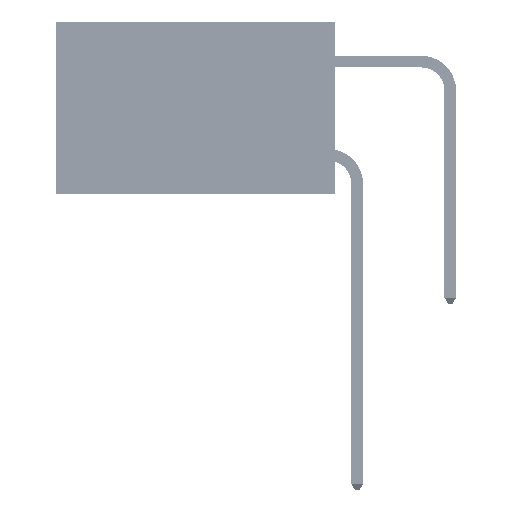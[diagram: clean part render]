
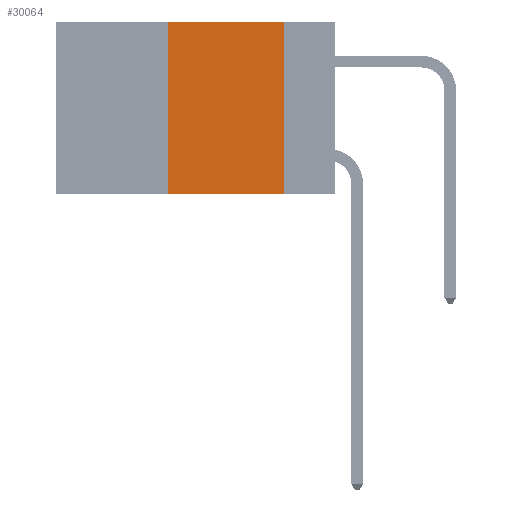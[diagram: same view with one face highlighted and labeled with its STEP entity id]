
A CAD part, left-side view. The second image highlights one B-rep face of the part: STEP entity #30064.
In plain terms, the highlighted planar face has unit normal (-1, 0, 0).
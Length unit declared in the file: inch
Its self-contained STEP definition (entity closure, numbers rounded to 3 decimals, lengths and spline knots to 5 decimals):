
#1715 = VECTOR ( 'NONE', #19208, 39.37008 ) ;
#3012 = ORIENTED_EDGE ( 'NONE', *, *, #25037, .F. ) ;
#3068 = VECTOR ( 'NONE', #46122, 39.37008 ) ;
#3172 = LINE ( 'NONE', #52972, #34026 ) ;
#4730 = CARTESIAN_POINT ( 'NONE',  ( 0., 0.36, -0.37 ) ) ;
#5806 = DIRECTION ( 'NONE',  ( 0., -1., 0. ) ) ;
#8840 = EDGE_CURVE ( 'NONE', #35283, #36188, #25039, .T. ) ;
#9728 = DIRECTION ( 'NONE',  ( 1., 0., 0. ) ) ;
#13842 = PLANE ( 'NONE',  #36107 ) ;
#15502 = DIRECTION ( 'NONE',  ( 0., 0., -1. ) ) ;
#17954 = FACE_OUTER_BOUND ( 'NONE', #26679, .T. ) ;
#19208 = DIRECTION ( 'NONE',  ( 0., 0., 1. ) ) ;
#19419 = VERTEX_POINT ( 'NONE', #4730 ) ;
#22518 = LINE ( 'NONE', #51791, #1715 ) ;
#25037 = EDGE_CURVE ( 'NONE', #36188, #25665, #3172, .T. ) ;
#25039 = LINE ( 'NONE', #45303, #3068 ) ;
#25665 = VERTEX_POINT ( 'NONE', #37783 ) ;
#26409 = DIRECTION ( 'NONE',  ( 0., 0., -1. ) ) ;
#26596 = LINE ( 'NONE', #43300, #51174 ) ;
#26679 = EDGE_LOOP ( 'NONE', ( #3012, #34992, #41696, #34749 ) ) ;
#30064 = ADVANCED_FACE ( 'NONE', ( #17954 ), #13842, .F. ) ;
#30493 = CARTESIAN_POINT ( 'NONE',  ( 0., 0.6, 0. ) ) ;
#30561 = CARTESIAN_POINT ( 'NONE',  ( 0., 0.11, 0. ) ) ;
#34026 = VECTOR ( 'NONE', #15502, 39.37008 ) ;
#34749 = ORIENTED_EDGE ( 'NONE', *, *, #52347, .T. ) ;
#34992 = ORIENTED_EDGE ( 'NONE', *, *, #8840, .F. ) ;
#35283 = VERTEX_POINT ( 'NONE', #46899 ) ;
#36107 = AXIS2_PLACEMENT_3D ( 'NONE', #30493, #9728, #26409 ) ;
#36188 = VERTEX_POINT ( 'NONE', #30561 ) ;
#37783 = CARTESIAN_POINT ( 'NONE',  ( 0., 0.11, -0.37 ) ) ;
#41696 = ORIENTED_EDGE ( 'NONE', *, *, #44122, .F. ) ;
#43300 = CARTESIAN_POINT ( 'NONE',  ( 0., 0.6, -0.37 ) ) ;
#44122 = EDGE_CURVE ( 'NONE', #19419, #35283, #22518, .T. ) ;
#45303 = CARTESIAN_POINT ( 'NONE',  ( 0., 0.6, 0. ) ) ;
#46122 = DIRECTION ( 'NONE',  ( 0., -1., 0. ) ) ;
#46899 = CARTESIAN_POINT ( 'NONE',  ( 0., 0.36, 0. ) ) ;
#51174 = VECTOR ( 'NONE', #5806, 39.37008 ) ;
#51791 = CARTESIAN_POINT ( 'NONE',  ( 0., 0.36, 0. ) ) ;
#52347 = EDGE_CURVE ( 'NONE', #19419, #25665, #26596, .T. ) ;
#52972 = CARTESIAN_POINT ( 'NONE',  ( 0., 0.11, 0. ) ) ;
